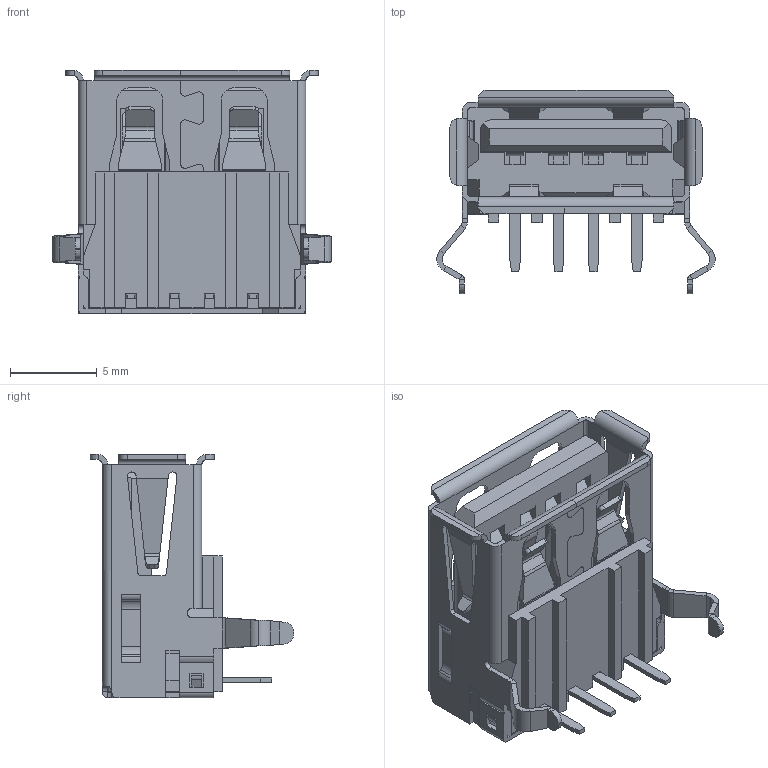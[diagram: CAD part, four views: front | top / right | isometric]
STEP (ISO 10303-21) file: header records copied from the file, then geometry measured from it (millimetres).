
FILE_DESCRIPTION (( 'STEP AP214' ), '1' );
FILE_NAME ('690A104-123-021.STEP', '2021-01-13T20:34:15', ( '' ), ( '' ), 'SwSTEP 2.0', 'SolidWorks 2020', '' );
FILE_SCHEMA (( 'AUTOMOTIVE_DESIGN' ));
Length unit declared in the file: millimetre
Products named in the file (4): Shell 690A104-X23-02X; Contact 690A104-X23-02X; Insulator 690A104-X23-02X_Black; 690A104-123-021
Assembly tree (6 placements, depth 2):
  690A104-123-021
    Insulator 690A104-X23-02X_Black
    Contact 690A104-X23-02X  x4
    Shell 690A104-X23-02X
Bounding box: 16 x 11.7 x 14 mm (x, y, z)
Volume: 576.4 mm3; surface area: 2131.2 mm2
Topology: 6 solids, 6 shells, 869 faces, 2476 edges, 1594 vertices
Faces by surface type: plane 656, cylinder 187, bspline 26
Entity records: 23252 total; most frequent: CARTESIAN_POINT 5051, ORIENTED_EDGE 3954, DIRECTION 3495, EDGE_CURVE 1977, VECTOR 1597, LINE 1597, VERTEX_POINT 1264, AXIS2_PLACEMENT_3D 949
